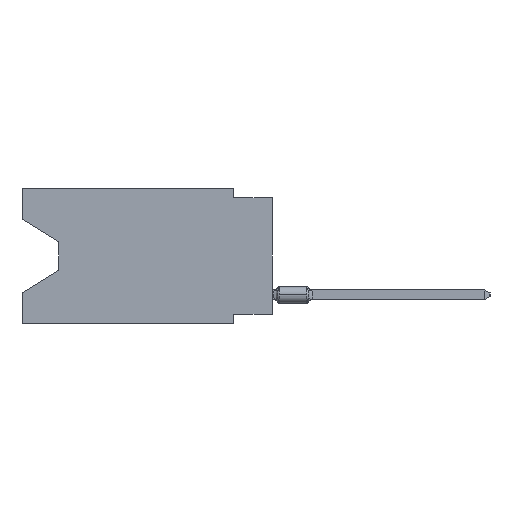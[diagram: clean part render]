
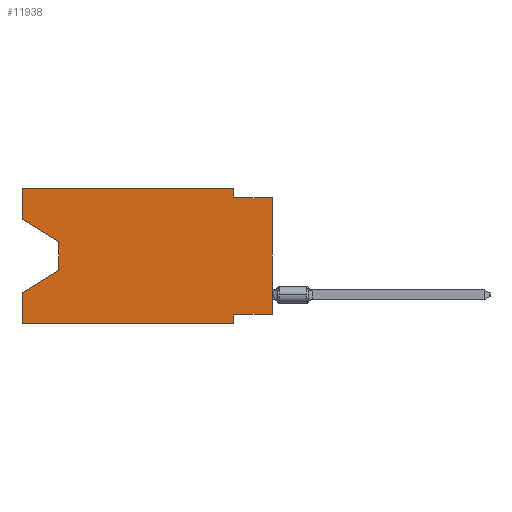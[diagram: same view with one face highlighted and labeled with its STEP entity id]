
A CAD part, left-side view. The second image highlights one B-rep face of the part: STEP entity #11938.
In plain terms, the highlighted planar face has unit normal (-1, 0, 0).
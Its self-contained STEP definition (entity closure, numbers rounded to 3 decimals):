
#189 = LINE ( 'NONE', #22819, #11602 ) ;
#845 = EDGE_CURVE ( 'NONE', #2221, #32230, #10887, .T. ) ;
#1382 = EDGE_CURVE ( 'NONE', #8709, #8653, #13822, .T. ) ;
#1613 = ORIENTED_EDGE ( 'NONE', *, *, #32848, .T. ) ;
#1880 = DIRECTION ( 'NONE',  ( 0., 0.855, -0.519 ) ) ;
#2221 = VERTEX_POINT ( 'NONE', #35366 ) ;
#2241 = CARTESIAN_POINT ( 'NONE',  ( 0., 2.54, -0.635 ) ) ;
#2329 = LINE ( 'NONE', #13657, #9405 ) ;
#2813 = VECTOR ( 'NONE', #16792, 1000. ) ;
#3484 = EDGE_CURVE ( 'NONE', #27087, #7066, #24997, .T. ) ;
#3958 = VECTOR ( 'NONE', #29770, 1000. ) ;
#4566 = CARTESIAN_POINT ( 'NONE',  ( 0., 16.383, -2.038 ) ) ;
#4739 = CARTESIAN_POINT ( 'NONE',  ( 0., 0., -0.635 ) ) ;
#4759 = LINE ( 'NONE', #4566, #33552 ) ;
#4959 = ORIENTED_EDGE ( 'NONE', *, *, #21293, .F. ) ;
#4979 = ORIENTED_EDGE ( 'NONE', *, *, #1382, .F. ) ;
#5141 = VECTOR ( 'NONE', #7624, 1000. ) ;
#5305 = CARTESIAN_POINT ( 'NONE',  ( 0., 2.54, -8.89 ) ) ;
#5857 = CARTESIAN_POINT ( 'NONE',  ( 0., 2.54, -8.89 ) ) ;
#6004 = EDGE_CURVE ( 'NONE', #17394, #15008, #31461, .T. ) ;
#6960 = VERTEX_POINT ( 'NONE', #23209 ) ;
#7025 = CARTESIAN_POINT ( 'NONE',  ( 0., 0., -8.255 ) ) ;
#7066 = VERTEX_POINT ( 'NONE', #21675 ) ;
#7081 = CARTESIAN_POINT ( 'NONE',  ( 0., 13.97, -5.385 ) ) ;
#7113 = CARTESIAN_POINT ( 'NONE',  ( 0., 13.97, -5.385 ) ) ;
#7624 = DIRECTION ( 'NONE',  ( 0., -1., 0. ) ) ;
#8405 = EDGE_LOOP ( 'NONE', ( #14350, #28206, #18787, #4979, #1613, #14196, #4959, #12072, #29723, #34576, #33743, #13593 ) ) ;
#8531 = EDGE_CURVE ( 'NONE', #35458, #2221, #4759, .T. ) ;
#8653 = VERTEX_POINT ( 'NONE', #13853 ) ;
#8709 = VERTEX_POINT ( 'NONE', #10878 ) ;
#8826 = AXIS2_PLACEMENT_3D ( 'NONE', #28929, #31702, #31538 ) ;
#9405 = VECTOR ( 'NONE', #35728, 1000. ) ;
#10680 = DIRECTION ( 'NONE',  ( 0., -1., 0. ) ) ;
#10712 = CARTESIAN_POINT ( 'NONE',  ( 0., 13.97, -3.505 ) ) ;
#10878 = CARTESIAN_POINT ( 'NONE',  ( 0., 16.383, -8.89 ) ) ;
#10887 = LINE ( 'NONE', #10712, #27096 ) ;
#11247 = DIRECTION ( 'NONE',  ( 0., 0., -1. ) ) ;
#11602 = VECTOR ( 'NONE', #34135, 1000. ) ;
#11938 = ADVANCED_FACE ( 'NONE', ( #19343 ), #24920, .F. ) ;
#12072 = ORIENTED_EDGE ( 'NONE', *, *, #30755, .T. ) ;
#13593 = ORIENTED_EDGE ( 'NONE', *, *, #35615, .F. ) ;
#13657 = CARTESIAN_POINT ( 'NONE',  ( 0., 16.383, 0. ) ) ;
#13822 = LINE ( 'NONE', #33857, #2813 ) ;
#13853 = CARTESIAN_POINT ( 'NONE',  ( 0., 16.383, -6.852 ) ) ;
#14196 = ORIENTED_EDGE ( 'NONE', *, *, #6004, .F. ) ;
#14240 = DIRECTION ( 'NONE',  ( 0., -1., 0. ) ) ;
#14350 = ORIENTED_EDGE ( 'NONE', *, *, #8531, .T. ) ;
#15008 = VERTEX_POINT ( 'NONE', #5305 ) ;
#15071 = LINE ( 'NONE', #20640, #31428 ) ;
#15916 = DIRECTION ( 'NONE',  ( 0., 0., -1. ) ) ;
#16525 = LINE ( 'NONE', #18744, #5141 ) ;
#16792 = DIRECTION ( 'NONE',  ( 0., 0., 1. ) ) ;
#17394 = VERTEX_POINT ( 'NONE', #27584 ) ;
#18471 = CARTESIAN_POINT ( 'NONE',  ( 0., 0., 0. ) ) ;
#18502 = DIRECTION ( 'NONE',  ( 0., -0.855, -0.519 ) ) ;
#18744 = CARTESIAN_POINT ( 'NONE',  ( 0., 16.383, -8.89 ) ) ;
#18787 = ORIENTED_EDGE ( 'NONE', *, *, #23462, .T. ) ;
#18931 = CARTESIAN_POINT ( 'NONE',  ( 0., 16.383, 0. ) ) ;
#19343 = FACE_OUTER_BOUND ( 'NONE', #8405, .T. ) ;
#19989 = VECTOR ( 'NONE', #10680, 1000. ) ;
#20036 = VERTEX_POINT ( 'NONE', #7025 ) ;
#20640 = CARTESIAN_POINT ( 'NONE',  ( 0., 2.54, 0. ) ) ;
#20890 = LINE ( 'NONE', #18471, #3958 ) ;
#21293 = EDGE_CURVE ( 'NONE', #20036, #17394, #189, .T. ) ;
#21419 = VECTOR ( 'NONE', #1880, 1000. ) ;
#21675 = CARTESIAN_POINT ( 'NONE',  ( 0., 2.54, 0. ) ) ;
#22599 = EDGE_CURVE ( 'NONE', #7066, #23619, #15071, .T. ) ;
#22819 = CARTESIAN_POINT ( 'NONE',  ( 0., 0., -8.255 ) ) ;
#23209 = CARTESIAN_POINT ( 'NONE',  ( 0., 0., -0.635 ) ) ;
#23462 = EDGE_CURVE ( 'NONE', #32230, #8653, #27303, .T. ) ;
#23619 = VERTEX_POINT ( 'NONE', #2241 ) ;
#24920 = PLANE ( 'NONE',  #8826 ) ;
#24997 = LINE ( 'NONE', #27967, #25609 ) ;
#25609 = VECTOR ( 'NONE', #14240, 1000. ) ;
#26280 = CARTESIAN_POINT ( 'NONE',  ( 0., 16.383, -2.038 ) ) ;
#27087 = VERTEX_POINT ( 'NONE', #18931 ) ;
#27096 = VECTOR ( 'NONE', #15916, 1000. ) ;
#27303 = LINE ( 'NONE', #7081, #21419 ) ;
#27584 = CARTESIAN_POINT ( 'NONE',  ( 0., 2.54, -8.255 ) ) ;
#27967 = CARTESIAN_POINT ( 'NONE',  ( 0., 16.383, 0. ) ) ;
#28206 = ORIENTED_EDGE ( 'NONE', *, *, #845, .T. ) ;
#28929 = CARTESIAN_POINT ( 'NONE',  ( 0., 16.383, 0. ) ) ;
#28988 = DIRECTION ( 'NONE',  ( 0., 0., -1. ) ) ;
#29723 = ORIENTED_EDGE ( 'NONE', *, *, #33294, .F. ) ;
#29770 = DIRECTION ( 'NONE',  ( 0., 0., 1. ) ) ;
#29827 = VECTOR ( 'NONE', #11247, 1000. ) ;
#30144 = LINE ( 'NONE', #4739, #19989 ) ;
#30755 = EDGE_CURVE ( 'NONE', #20036, #6960, #20890, .T. ) ;
#31428 = VECTOR ( 'NONE', #28988, 1000. ) ;
#31461 = LINE ( 'NONE', #5857, #29827 ) ;
#31538 = DIRECTION ( 'NONE',  ( 0., 0., -1. ) ) ;
#31702 = DIRECTION ( 'NONE',  ( 1., 0., 0. ) ) ;
#32230 = VERTEX_POINT ( 'NONE', #7113 ) ;
#32848 = EDGE_CURVE ( 'NONE', #8709, #15008, #16525, .T. ) ;
#33294 = EDGE_CURVE ( 'NONE', #23619, #6960, #30144, .T. ) ;
#33552 = VECTOR ( 'NONE', #18502, 1000. ) ;
#33743 = ORIENTED_EDGE ( 'NONE', *, *, #3484, .F. ) ;
#33857 = CARTESIAN_POINT ( 'NONE',  ( 0., 16.383, 0. ) ) ;
#34135 = DIRECTION ( 'NONE',  ( 0., 1., 0. ) ) ;
#34576 = ORIENTED_EDGE ( 'NONE', *, *, #22599, .F. ) ;
#35366 = CARTESIAN_POINT ( 'NONE',  ( 0., 13.97, -3.505 ) ) ;
#35458 = VERTEX_POINT ( 'NONE', #26280 ) ;
#35615 = EDGE_CURVE ( 'NONE', #35458, #27087, #2329, .T. ) ;
#35728 = DIRECTION ( 'NONE',  ( 0., 0., 1. ) ) ;
